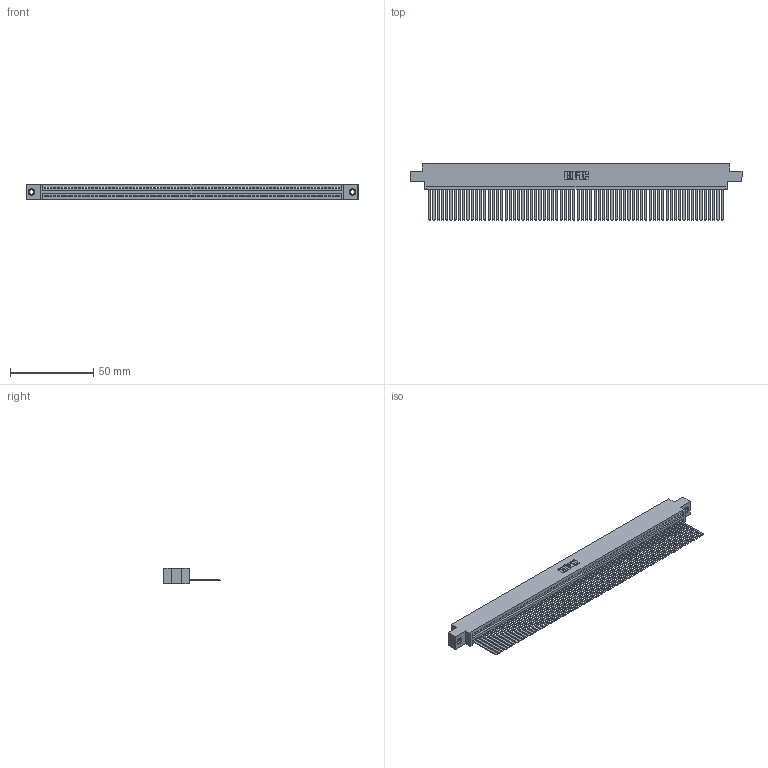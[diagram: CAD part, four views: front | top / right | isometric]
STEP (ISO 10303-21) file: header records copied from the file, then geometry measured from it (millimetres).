
FILE_DESCRIPTION (( 'STEP AP203' ), '1' );
FILE_NAME ('345-070-544-607.STEP', '2018-10-01T09:09:20', ( '' ), ( '' ), 'SwSTEP 2.0', 'SolidWorks 2016', '' );
FILE_SCHEMA (( 'CONFIG_CONTROL_DESIGN' ));
Length unit declared in the file: inch
Products named in the file (4): 345-070-544-607; 345-250-001_345-250-005-103; 345 Part_0.170 Offset - 0.156 Dia-TI; 345-292-001_345-293-144
Assembly tree (73 placements, depth 2):
  345-070-544-607
    345 Part_0.170 Offset - 0.156 Dia-TI
    345-292-001_345-293-144  x70
    345-250-001_345-250-005-103  x2
Bounding box: 199.01 x 33.96 x 9.4 mm (x, y, z)
Volume: 19815.2 mm3; surface area: 29306.1 mm2
Topology: 73 solids, 73 shells, 3830 faces, 11549 edges, 7598 vertices
Faces by surface type: plane 2636, cylinder 1178, cone 12, torus 4
Entity records: 50048 total; most frequent: CARTESIAN_POINT 8649, ORIENTED_EDGE 8646, DIRECTION 7537, EDGE_CURVE 4323, LINE 3895, VECTOR 3895, VERTEX_POINT 2876, AXIS2_PLACEMENT_3D 1821
